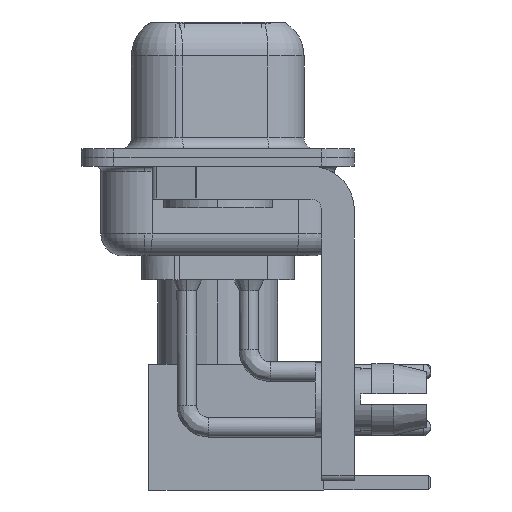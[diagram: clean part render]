
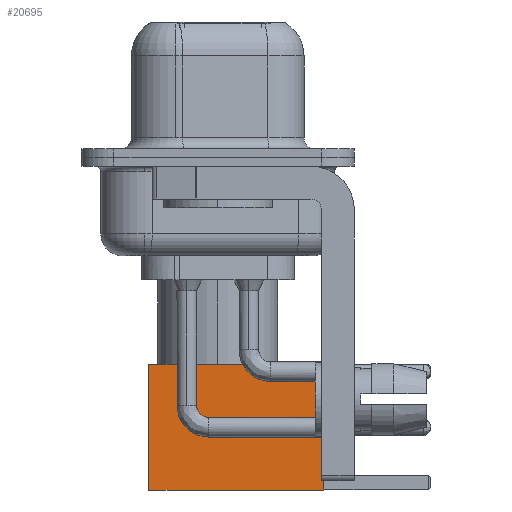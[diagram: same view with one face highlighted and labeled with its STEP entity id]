
A CAD part, left-side view. The second image highlights one B-rep face of the part: STEP entity #20695.
In plain terms, the highlighted face is planar.
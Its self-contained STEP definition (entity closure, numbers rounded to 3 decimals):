
#67 = LINE ( 'NONE', #17886, #11825 ) ;
#402 = EDGE_CURVE ( 'NONE', #18345, #24412, #12615, .T. ) ;
#735 = DIRECTION ( 'NONE',  ( -1., 0., 0. ) ) ;
#1691 = VECTOR ( 'NONE', #18877, 1000. ) ;
#2048 = CARTESIAN_POINT ( 'NONE',  ( -2.875, 2.875, 0. ) ) ;
#2163 = ORIENTED_EDGE ( 'NONE', *, *, #14728, .F. ) ;
#2546 = ORIENTED_EDGE ( 'NONE', *, *, #402, .T. ) ;
#4232 = LINE ( 'NONE', #2048, #23389 ) ;
#4260 = EDGE_LOOP ( 'NONE', ( #21078, #2546, #2163, #19504 ) ) ;
#4527 = DIRECTION ( 'NONE',  ( 0., 0., 1. ) ) ;
#4913 = CARTESIAN_POINT ( 'NONE',  ( 0., 2.875, 0. ) ) ;
#10436 = FACE_OUTER_BOUND ( 'NONE', #4260, .T. ) ;
#10868 = VERTEX_POINT ( 'NONE', #21607 ) ;
#11825 = VECTOR ( 'NONE', #13790, 1000. ) ;
#12369 = DIRECTION ( 'NONE',  ( 0., 1., 0. ) ) ;
#12615 = LINE ( 'NONE', #4913, #1691 ) ;
#12763 = CARTESIAN_POINT ( 'NONE',  ( -2.875, 2.875, 0. ) ) ;
#13790 = DIRECTION ( 'NONE',  ( 0., 0., -1. ) ) ;
#14033 = PLANE ( 'NONE',  #19132 ) ;
#14728 = EDGE_CURVE ( 'NONE', #23265, #24412, #4232, .T. ) ;
#14828 = EDGE_CURVE ( 'NONE', #10868, #23265, #22040, .T. ) ;
#15082 = CARTESIAN_POINT ( 'NONE',  ( 2.875, 2.875, 0. ) ) ;
#16247 = CARTESIAN_POINT ( 'NONE',  ( 0., 2.875, 8. ) ) ;
#16381 = CARTESIAN_POINT ( 'NONE',  ( -2.875, 2.875, 8. ) ) ;
#17699 = DIRECTION ( 'NONE',  ( 0., 0., -1. ) ) ;
#17886 = CARTESIAN_POINT ( 'NONE',  ( 2.875, 2.875, 0. ) ) ;
#18345 = VERTEX_POINT ( 'NONE', #15082 ) ;
#18877 = DIRECTION ( 'NONE',  ( -1., 0., 0. ) ) ;
#19132 = AXIS2_PLACEMENT_3D ( 'NONE', #21844, #12369, #4527 ) ;
#19504 = ORIENTED_EDGE ( 'NONE', *, *, #14828, .F. ) ;
#20695 = ADVANCED_FACE ( 'NONE', ( #10436 ), #14033, .T. ) ;
#21078 = ORIENTED_EDGE ( 'NONE', *, *, #21434, .T. ) ;
#21434 = EDGE_CURVE ( 'NONE', #10868, #18345, #67, .T. ) ;
#21607 = CARTESIAN_POINT ( 'NONE',  ( 2.875, 2.875, 8. ) ) ;
#21844 = CARTESIAN_POINT ( 'NONE',  ( 2.875, 2.875, 0. ) ) ;
#22040 = LINE ( 'NONE', #16247, #24604 ) ;
#23265 = VERTEX_POINT ( 'NONE', #16381 ) ;
#23389 = VECTOR ( 'NONE', #17699, 1000. ) ;
#24412 = VERTEX_POINT ( 'NONE', #12763 ) ;
#24604 = VECTOR ( 'NONE', #735, 1000. ) ;
